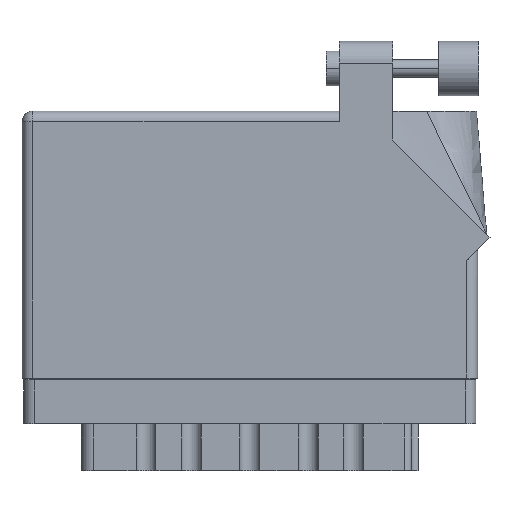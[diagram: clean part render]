
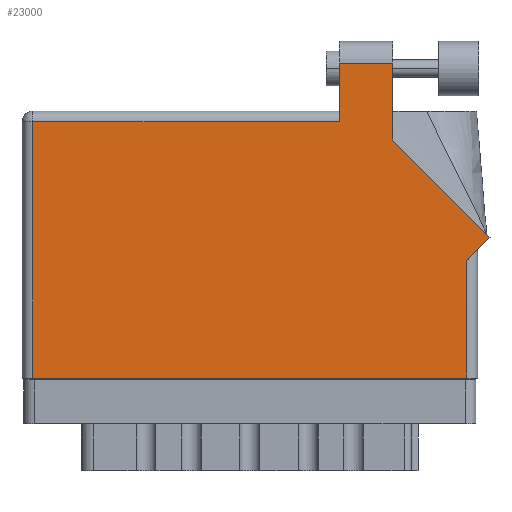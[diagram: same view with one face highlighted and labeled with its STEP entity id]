
A CAD part, front view. The second image highlights one B-rep face of the part: STEP entity #23000.
In plain terms, the highlighted face is planar.
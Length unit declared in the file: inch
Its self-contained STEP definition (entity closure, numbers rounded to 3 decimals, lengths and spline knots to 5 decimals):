
#540 = AXIS2_PLACEMENT_3D ( 'NONE', #46919, #31679, #17074 ) ;
#1000 = ORIENTED_EDGE ( 'NONE', *, *, #19457, .T. ) ;
#1336 = PLANE ( 'NONE',  #540 ) ;
#2351 = DIRECTION ( 'NONE',  ( 0., 1., 0. ) ) ;
#2353 = ORIENTED_EDGE ( 'NONE', *, *, #29036, .T. ) ;
#2618 = DIRECTION ( 'NONE',  ( -0.707, 0.707, 0. ) ) ;
#3359 = VECTOR ( 'NONE', #39213, 39.37008 ) ;
#3715 = VECTOR ( 'NONE', #35128, 39.37008 ) ;
#4842 = CARTESIAN_POINT ( 'NONE',  ( 1.819, 1.805, 0. ) ) ;
#5910 = LINE ( 'NONE', #43491, #27231 ) ;
#7606 = CARTESIAN_POINT ( 'NONE',  ( 0., 0., 0. ) ) ;
#7670 = VECTOR ( 'NONE', #35688, 39.37008 ) ;
#8364 = EDGE_CURVE ( 'NONE', #10053, #44371, #32576, .T. ) ;
#8434 = ORIENTED_EDGE ( 'NONE', *, *, #12848, .T. ) ;
#8614 = LINE ( 'NONE', #7606, #37624 ) ;
#9256 = CARTESIAN_POINT ( 'NONE',  ( 1.819, 1.805, 0. ) ) ;
#10053 = VERTEX_POINT ( 'NONE', #9256 ) ;
#10929 = ORIENTED_EDGE ( 'NONE', *, *, #35901, .T. ) ;
#10979 = VERTEX_POINT ( 'NONE', #13218 ) ;
#11702 = CARTESIAN_POINT ( 'NONE',  ( 2.126, 1.36442, 0. ) ) ;
#12848 = EDGE_CURVE ( 'NONE', #24944, #10979, #28987, .T. ) ;
#12929 = LINE ( 'NONE', #49032, #21796 ) ;
#13218 = CARTESIAN_POINT ( 'NONE',  ( 0.062, 0., 0. ) ) ;
#14715 = CARTESIAN_POINT ( 'NONE',  ( 2.126, 1.805, 0. ) ) ;
#15217 = VERTEX_POINT ( 'NONE', #14715 ) ;
#15938 = ORIENTED_EDGE ( 'NONE', *, *, #25264, .T. ) ;
#16140 = VECTOR ( 'NONE', #17117, 39.37008 ) ;
#16309 = DIRECTION ( 'NONE',  ( 0., -1., 0. ) ) ;
#16706 = CARTESIAN_POINT ( 'NONE',  ( 0.062, 1.468, 0. ) ) ;
#17074 = DIRECTION ( 'NONE',  ( -1., 0., 0. ) ) ;
#17117 = DIRECTION ( 'NONE',  ( 0., 1., 0. ) ) ;
#17708 = FACE_OUTER_BOUND ( 'NONE', #23376, .T. ) ;
#18371 = DIRECTION ( 'NONE',  ( 0.707, 0.707, 0. ) ) ;
#19273 = CARTESIAN_POINT ( 'NONE',  ( 2.55, 0., 0. ) ) ;
#19457 = EDGE_CURVE ( 'NONE', #44371, #24944, #25898, .T. ) ;
#19964 = VERTEX_POINT ( 'NONE', #19273 ) ;
#21796 = VECTOR ( 'NONE', #18371, 39.37008 ) ;
#23000 = ADVANCED_FACE ( 'NONE', ( #17708 ), #1336, .F. ) ;
#23376 = EDGE_LOOP ( 'NONE', ( #28745, #10929, #45165, #1000, #8434, #15938, #35738, #2353, #44559 ) ) ;
#23799 = CARTESIAN_POINT ( 'NONE',  ( 0., 1.468, 0. ) ) ;
#24591 = CARTESIAN_POINT ( 'NONE',  ( 2.126, 1.36442, 0. ) ) ;
#24944 = VERTEX_POINT ( 'NONE', #16706 ) ;
#25264 = EDGE_CURVE ( 'NONE', #10979, #19964, #8614, .T. ) ;
#25898 = LINE ( 'NONE', #23799, #3359 ) ;
#26814 = LINE ( 'NONE', #4842, #3715 ) ;
#27231 = VECTOR ( 'NONE', #2351, 39.37008 ) ;
#28167 = EDGE_CURVE ( 'NONE', #19964, #40385, #5910, .T. ) ;
#28745 = ORIENTED_EDGE ( 'NONE', *, *, #46012, .T. ) ;
#28920 = EDGE_CURVE ( 'NONE', #47900, #41636, #32510, .T. ) ;
#28987 = LINE ( 'NONE', #43669, #7670 ) ;
#29036 = EDGE_CURVE ( 'NONE', #40385, #47900, #12929, .T. ) ;
#30192 = CARTESIAN_POINT ( 'NONE',  ( 2.55, 0.675, 0. ) ) ;
#31679 = DIRECTION ( 'NONE',  ( 0., 0., -1. ) ) ;
#31735 = CARTESIAN_POINT ( 'NONE',  ( 1.819, 1.53, 0. ) ) ;
#32510 = LINE ( 'NONE', #32626, #42557 ) ;
#32576 = LINE ( 'NONE', #31735, #37894 ) ;
#32626 = CARTESIAN_POINT ( 'NONE',  ( 2.68271, 0.80771, 0. ) ) ;
#35128 = DIRECTION ( 'NONE',  ( -1., 0., 0. ) ) ;
#35688 = DIRECTION ( 'NONE',  ( 0., -1., 0. ) ) ;
#35738 = ORIENTED_EDGE ( 'NONE', *, *, #28167, .T. ) ;
#35901 = EDGE_CURVE ( 'NONE', #15217, #10053, #26814, .T. ) ;
#37624 = VECTOR ( 'NONE', #42215, 39.37008 ) ;
#37894 = VECTOR ( 'NONE', #16309, 39.37008 ) ;
#39213 = DIRECTION ( 'NONE',  ( -1., 0., 0. ) ) ;
#40123 = CARTESIAN_POINT ( 'NONE',  ( 1.819, 1.468, 0. ) ) ;
#40385 = VERTEX_POINT ( 'NONE', #30192 ) ;
#41622 = CARTESIAN_POINT ( 'NONE',  ( 2.68271, 0.80771, 0. ) ) ;
#41636 = VERTEX_POINT ( 'NONE', #11702 ) ;
#42215 = DIRECTION ( 'NONE',  ( 1., 0., 0. ) ) ;
#42557 = VECTOR ( 'NONE', #2618, 39.37008 ) ;
#43491 = CARTESIAN_POINT ( 'NONE',  ( 2.55, 0.737, 0. ) ) ;
#43669 = CARTESIAN_POINT ( 'NONE',  ( 0.062, 0., 0. ) ) ;
#44371 = VERTEX_POINT ( 'NONE', #40123 ) ;
#44559 = ORIENTED_EDGE ( 'NONE', *, *, #28920, .T. ) ;
#45165 = ORIENTED_EDGE ( 'NONE', *, *, #8364, .T. ) ;
#46012 = EDGE_CURVE ( 'NONE', #41636, #15217, #47594, .T. ) ;
#46919 = CARTESIAN_POINT ( 'NONE',  ( 0., 1.53, 0. ) ) ;
#47594 = LINE ( 'NONE', #24591, #16140 ) ;
#47900 = VERTEX_POINT ( 'NONE', #41622 ) ;
#49032 = CARTESIAN_POINT ( 'NONE',  ( 2.612, 0.737, 0. ) ) ;
